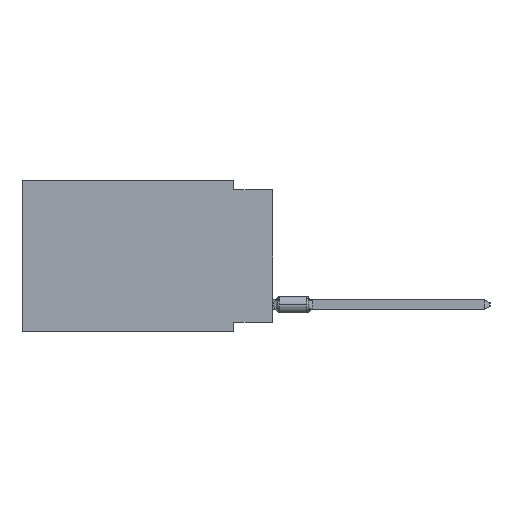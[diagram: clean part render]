
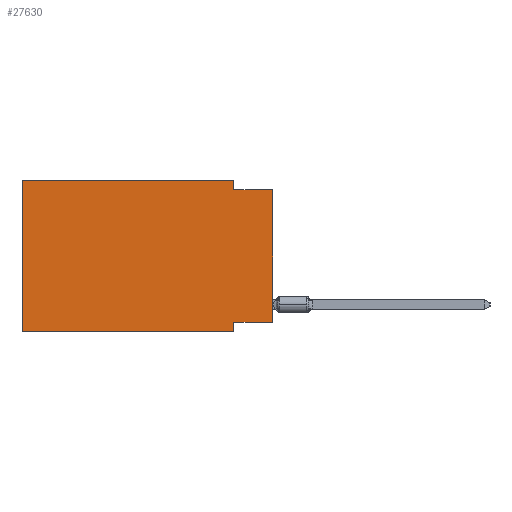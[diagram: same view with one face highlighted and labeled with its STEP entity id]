
A CAD part, left-side view. The second image highlights one B-rep face of the part: STEP entity #27630.
In plain terms, the highlighted planar face has unit normal (-1, 0, 0).
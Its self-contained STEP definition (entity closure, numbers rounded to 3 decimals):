
#1667 = DIRECTION ( 'NONE',  ( 0., 0., -1. ) ) ;
#1777 = LINE ( 'NONE', #2137, #13067 ) ;
#2137 = CARTESIAN_POINT ( 'NONE',  ( 0., 0., -0.635 ) ) ;
#2554 = LINE ( 'NONE', #12873, #35550 ) ;
#3718 = ORIENTED_EDGE ( 'NONE', *, *, #12509, .F. ) ;
#5220 = VECTOR ( 'NONE', #1667, 1000. ) ;
#5602 = CARTESIAN_POINT ( 'NONE',  ( 0., 2.54, -9.271 ) ) ;
#6646 = LINE ( 'NONE', #18352, #5220 ) ;
#8292 = EDGE_CURVE ( 'NONE', #44855, #22464, #1777, .T. ) ;
#8461 = VECTOR ( 'NONE', #30302, 1000. ) ;
#8953 = CARTESIAN_POINT ( 'NONE',  ( 0., 16.383, 0. ) ) ;
#9597 = CARTESIAN_POINT ( 'NONE',  ( 0., 16.383, -9.906 ) ) ;
#9708 = EDGE_CURVE ( 'NONE', #28126, #53071, #38801, .T. ) ;
#10386 = PLANE ( 'NONE',  #10905 ) ;
#10492 = LINE ( 'NONE', #53865, #46585 ) ;
#10905 = AXIS2_PLACEMENT_3D ( 'NONE', #48428, #32101, #38141 ) ;
#12101 = DIRECTION ( 'NONE',  ( 0., -1., 0. ) ) ;
#12509 = EDGE_CURVE ( 'NONE', #53071, #44855, #6646, .T. ) ;
#12873 = CARTESIAN_POINT ( 'NONE',  ( 0., 2.54, -9.906 ) ) ;
#13067 = VECTOR ( 'NONE', #34516, 1000. ) ;
#13107 = CARTESIAN_POINT ( 'NONE',  ( 0., 2.54, -0.635 ) ) ;
#13233 = LINE ( 'NONE', #8953, #8461 ) ;
#13547 = CARTESIAN_POINT ( 'NONE',  ( 0., 16.383, -9.906 ) ) ;
#14777 = DIRECTION ( 'NONE',  ( 0., 0., 1. ) ) ;
#17818 = VERTEX_POINT ( 'NONE', #45240 ) ;
#18352 = CARTESIAN_POINT ( 'NONE',  ( 0., 2.54, 0. ) ) ;
#20362 = ORIENTED_EDGE ( 'NONE', *, *, #44204, .T. ) ;
#21754 = FACE_OUTER_BOUND ( 'NONE', #31774, .T. ) ;
#22464 = VERTEX_POINT ( 'NONE', #31393 ) ;
#25074 = EDGE_CURVE ( 'NONE', #26783, #28126, #13233, .T. ) ;
#26005 = ORIENTED_EDGE ( 'NONE', *, *, #35963, .F. ) ;
#26783 = VERTEX_POINT ( 'NONE', #9597 ) ;
#27064 = CARTESIAN_POINT ( 'NONE',  ( 0., 2.54, 0. ) ) ;
#27315 = VECTOR ( 'NONE', #28870, 1000. ) ;
#27630 = ADVANCED_FACE ( 'NONE', ( #21754 ), #10386, .F. ) ;
#28126 = VERTEX_POINT ( 'NONE', #63801 ) ;
#28870 = DIRECTION ( 'NONE',  ( 0., -1., 0. ) ) ;
#30302 = DIRECTION ( 'NONE',  ( 0., 0., 1. ) ) ;
#30611 = ORIENTED_EDGE ( 'NONE', *, *, #53463, .F. ) ;
#31393 = CARTESIAN_POINT ( 'NONE',  ( 0., 0., -0.635 ) ) ;
#31774 = EDGE_LOOP ( 'NONE', ( #20362, #38377, #3718, #56525, #63998, #51077, #26005, #30611 ) ) ;
#32101 = DIRECTION ( 'NONE',  ( 1., 0., 0. ) ) ;
#32324 = LINE ( 'NONE', #43354, #60011 ) ;
#32673 = DIRECTION ( 'NONE',  ( 0., 1., 0. ) ) ;
#33620 = EDGE_CURVE ( 'NONE', #26783, #17818, #67230, .T. ) ;
#34516 = DIRECTION ( 'NONE',  ( 0., -1., 0. ) ) ;
#35550 = VECTOR ( 'NONE', #45243, 1000. ) ;
#35963 = EDGE_CURVE ( 'NONE', #63007, #17818, #2554, .T. ) ;
#38141 = DIRECTION ( 'NONE',  ( 0., 0., -1. ) ) ;
#38377 = ORIENTED_EDGE ( 'NONE', *, *, #8292, .F. ) ;
#38801 = LINE ( 'NONE', #49441, #57466 ) ;
#42212 = CARTESIAN_POINT ( 'NONE',  ( 0., 0., -9.271 ) ) ;
#43354 = CARTESIAN_POINT ( 'NONE',  ( 0., 0., -9.271 ) ) ;
#44204 = EDGE_CURVE ( 'NONE', #52548, #22464, #10492, .T. ) ;
#44855 = VERTEX_POINT ( 'NONE', #13107 ) ;
#45240 = CARTESIAN_POINT ( 'NONE',  ( 0., 2.54, -9.906 ) ) ;
#45243 = DIRECTION ( 'NONE',  ( 0., 0., -1. ) ) ;
#46585 = VECTOR ( 'NONE', #14777, 1000. ) ;
#48428 = CARTESIAN_POINT ( 'NONE',  ( 0., 16.383, 0. ) ) ;
#49441 = CARTESIAN_POINT ( 'NONE',  ( 0., 16.383, 0. ) ) ;
#51077 = ORIENTED_EDGE ( 'NONE', *, *, #33620, .T. ) ;
#52548 = VERTEX_POINT ( 'NONE', #42212 ) ;
#53071 = VERTEX_POINT ( 'NONE', #27064 ) ;
#53463 = EDGE_CURVE ( 'NONE', #52548, #63007, #32324, .T. ) ;
#53865 = CARTESIAN_POINT ( 'NONE',  ( 0., 0., 0. ) ) ;
#56525 = ORIENTED_EDGE ( 'NONE', *, *, #9708, .F. ) ;
#57466 = VECTOR ( 'NONE', #12101, 1000. ) ;
#60011 = VECTOR ( 'NONE', #32673, 1000. ) ;
#63007 = VERTEX_POINT ( 'NONE', #5602 ) ;
#63801 = CARTESIAN_POINT ( 'NONE',  ( 0., 16.383, 0. ) ) ;
#63998 = ORIENTED_EDGE ( 'NONE', *, *, #25074, .F. ) ;
#67230 = LINE ( 'NONE', #13547, #27315 ) ;
